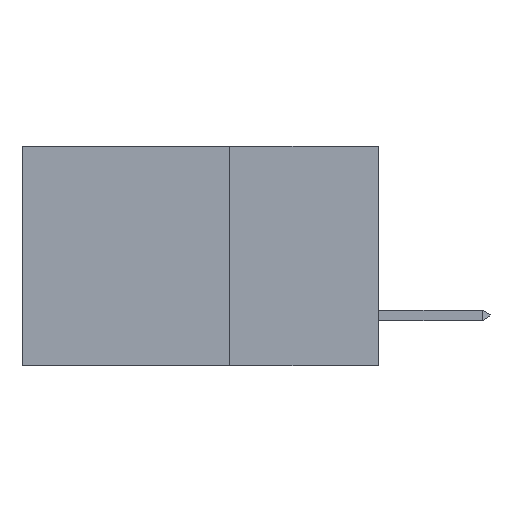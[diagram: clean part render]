
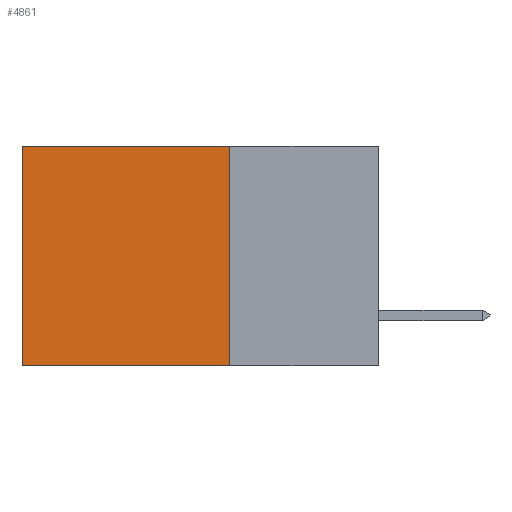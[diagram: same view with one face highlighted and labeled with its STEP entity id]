
A CAD part, left-side view. The second image highlights one B-rep face of the part: STEP entity #4861.
In plain terms, the highlighted planar face has unit normal (-1, 0, 0).
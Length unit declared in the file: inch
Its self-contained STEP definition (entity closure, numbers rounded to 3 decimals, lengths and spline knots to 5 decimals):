
#71 = VECTOR ( 'NONE', #11179, 39.37008 ) ;
#248 = DIRECTION ( 'NONE',  ( 1., 0., 0. ) ) ;
#643 = VECTOR ( 'NONE', #2888, 39.37008 ) ;
#687 = CARTESIAN_POINT ( 'NONE',  ( 0.298, 0.25, -0.37 ) ) ;
#822 = CARTESIAN_POINT ( 'NONE',  ( 0.298, 0.25, 0. ) ) ;
#1233 = VERTEX_POINT ( 'NONE', #4606 ) ;
#1641 = DIRECTION ( 'NONE',  ( 0., 0., -1. ) ) ;
#1960 = VECTOR ( 'NONE', #1641, 39.37008 ) ;
#2080 = LINE ( 'NONE', #3776, #11909 ) ;
#2133 = ORIENTED_EDGE ( 'NONE', *, *, #8196, .T. ) ;
#2371 = EDGE_LOOP ( 'NONE', ( #2133, #3744, #8700, #6888 ) ) ;
#2888 = DIRECTION ( 'NONE',  ( 0., 1., 0. ) ) ;
#3235 = DIRECTION ( 'NONE',  ( 0., 0., -1. ) ) ;
#3284 = CARTESIAN_POINT ( 'NONE',  ( 0.298, 0.6, 0. ) ) ;
#3332 = LINE ( 'NONE', #822, #643 ) ;
#3744 = ORIENTED_EDGE ( 'NONE', *, *, #9259, .F. ) ;
#3776 = CARTESIAN_POINT ( 'NONE',  ( 0.298, 0.25, -0.37 ) ) ;
#4606 = CARTESIAN_POINT ( 'NONE',  ( 0.298, 0.25, 0. ) ) ;
#4861 = ADVANCED_FACE ( 'NONE', ( #5327 ), #6434, .F. ) ;
#5327 = FACE_OUTER_BOUND ( 'NONE', #2371, .T. ) ;
#5399 = LINE ( 'NONE', #11854, #71 ) ;
#5771 = CARTESIAN_POINT ( 'NONE',  ( 0.298, 0.6, 0. ) ) ;
#6434 = PLANE ( 'NONE',  #9077 ) ;
#6888 = ORIENTED_EDGE ( 'NONE', *, *, #9521, .T. ) ;
#7872 = VERTEX_POINT ( 'NONE', #9120 ) ;
#8196 = EDGE_CURVE ( 'NONE', #12149, #7872, #11458, .T. ) ;
#8377 = EDGE_CURVE ( 'NONE', #1233, #9541, #5399, .T. ) ;
#8700 = ORIENTED_EDGE ( 'NONE', *, *, #8377, .F. ) ;
#9077 = AXIS2_PLACEMENT_3D ( 'NONE', #10241, #248, #3235 ) ;
#9120 = CARTESIAN_POINT ( 'NONE',  ( 0.298, 0.6, -0.37 ) ) ;
#9259 = EDGE_CURVE ( 'NONE', #9541, #7872, #2080, .T. ) ;
#9521 = EDGE_CURVE ( 'NONE', #1233, #12149, #3332, .T. ) ;
#9541 = VERTEX_POINT ( 'NONE', #687 ) ;
#10241 = CARTESIAN_POINT ( 'NONE',  ( 0.298, 0.25, 0. ) ) ;
#11179 = DIRECTION ( 'NONE',  ( 0., 0., -1. ) ) ;
#11458 = LINE ( 'NONE', #5771, #1960 ) ;
#11698 = DIRECTION ( 'NONE',  ( 0., 1., 0. ) ) ;
#11854 = CARTESIAN_POINT ( 'NONE',  ( 0.298, 0.25, 0. ) ) ;
#11909 = VECTOR ( 'NONE', #11698, 39.37008 ) ;
#12149 = VERTEX_POINT ( 'NONE', #3284 ) ;
